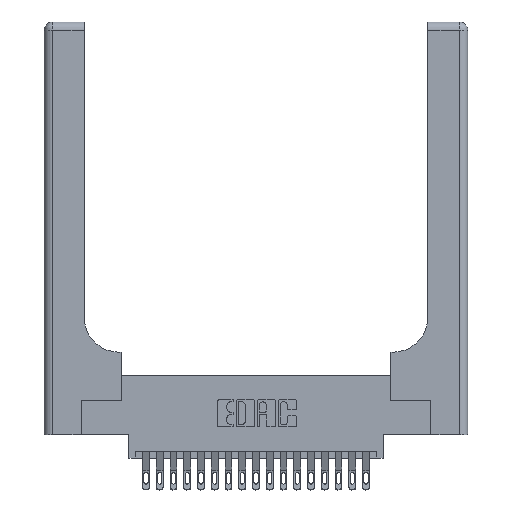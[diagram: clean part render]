
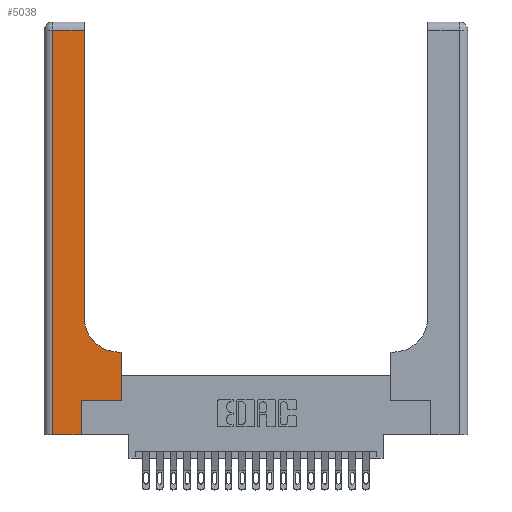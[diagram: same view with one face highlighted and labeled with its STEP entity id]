
A CAD part, top view. The second image highlights one B-rep face of the part: STEP entity #5038.
In plain terms, the highlighted planar face has unit normal (0, 0, 1).
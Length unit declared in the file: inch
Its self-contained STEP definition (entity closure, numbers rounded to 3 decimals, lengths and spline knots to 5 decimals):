
#271 = VERTEX_POINT ( 'NONE', #5505 ) ;
#707 = LINE ( 'NONE', #920, #3952 ) ;
#920 = CARTESIAN_POINT ( 'NONE',  ( 0., 2.94, 0.37 ) ) ;
#948 = LINE ( 'NONE', #12074, #3645 ) ;
#1036 = LINE ( 'NONE', #12148, #11002 ) ;
#1295 = CARTESIAN_POINT ( 'NONE',  ( 0.269, 0., 0.37 ) ) ;
#1308 = EDGE_CURVE ( 'NONE', #8733, #8761, #15321, .T. ) ;
#1400 = CIRCLE ( 'NONE', #7907, 0.25 ) ;
#1507 = CARTESIAN_POINT ( 'NONE',  ( 0.2915, 0.85, 0.37 ) ) ;
#1630 = ORIENTED_EDGE ( 'NONE', *, *, #9048, .T. ) ;
#2357 = DIRECTION ( 'NONE',  ( -1., 0., 0. ) ) ;
#2714 = VECTOR ( 'NONE', #3024, 39.37008 ) ;
#2720 = CARTESIAN_POINT ( 'NONE',  ( 0.5585, 0.6, 0.37 ) ) ;
#2778 = CARTESIAN_POINT ( 'NONE',  ( 0.269, 0.25, 0.37 ) ) ;
#2927 = CARTESIAN_POINT ( 'NONE',  ( 0.2915, 2.94, 0.37 ) ) ;
#3024 = DIRECTION ( 'NONE',  ( 0., 1., 0. ) ) ;
#3099 = VERTEX_POINT ( 'NONE', #20224 ) ;
#3645 = VECTOR ( 'NONE', #12151, 39.37008 ) ;
#3757 = DIRECTION ( 'NONE',  ( 1., 0., 0. ) ) ;
#3952 = VECTOR ( 'NONE', #19974, 39.37008 ) ;
#5038 = ADVANCED_FACE ( 'NONE', ( #20860 ), #10703, .F. ) ;
#5185 = DIRECTION ( 'NONE',  ( 0., 0., -1. ) ) ;
#5505 = CARTESIAN_POINT ( 'NONE',  ( 0.269, 0., 0.37 ) ) ;
#6190 = ORIENTED_EDGE ( 'NONE', *, *, #9986, .T. ) ;
#6917 = ORIENTED_EDGE ( 'NONE', *, *, #10793, .T. ) ;
#7112 = ORIENTED_EDGE ( 'NONE', *, *, #17414, .T. ) ;
#7198 = ORIENTED_EDGE ( 'NONE', *, *, #14333, .T. ) ;
#7817 = LINE ( 'NONE', #20428, #13221 ) ;
#7907 = AXIS2_PLACEMENT_3D ( 'NONE', #8858, #5185, #10287 ) ;
#8057 = ORIENTED_EDGE ( 'NONE', *, *, #1308, .T. ) ;
#8194 = AXIS2_PLACEMENT_3D ( 'NONE', #10933, #19510, #2357 ) ;
#8733 = VERTEX_POINT ( 'NONE', #13146 ) ;
#8761 = VERTEX_POINT ( 'NONE', #2720 ) ;
#8839 = VERTEX_POINT ( 'NONE', #1507 ) ;
#8858 = CARTESIAN_POINT ( 'NONE',  ( 0.5415, 0.85, 0.37 ) ) ;
#9048 = EDGE_CURVE ( 'NONE', #8839, #12609, #1036, .T. ) ;
#9986 = EDGE_CURVE ( 'NONE', #12609, #17768, #707, .T. ) ;
#10287 = DIRECTION ( 'NONE',  ( 1., 0., 0. ) ) ;
#10338 = ORIENTED_EDGE ( 'NONE', *, *, #17606, .T. ) ;
#10703 = PLANE ( 'NONE',  #8194 ) ;
#10793 = EDGE_CURVE ( 'NONE', #17768, #3099, #948, .T. ) ;
#10933 = CARTESIAN_POINT ( 'NONE',  ( 0., 3., 0.37 ) ) ;
#11002 = VECTOR ( 'NONE', #19029, 39.37008 ) ;
#11809 = VECTOR ( 'NONE', #13746, 39.37008 ) ;
#12074 = CARTESIAN_POINT ( 'NONE',  ( 0.06, 3., 0.37 ) ) ;
#12148 = CARTESIAN_POINT ( 'NONE',  ( 0.2915, 3., 0.37 ) ) ;
#12151 = DIRECTION ( 'NONE',  ( 0., -1., 0. ) ) ;
#12609 = VERTEX_POINT ( 'NONE', #2927 ) ;
#12983 = LINE ( 'NONE', #1295, #2714 ) ;
#13146 = CARTESIAN_POINT ( 'NONE',  ( 0.5585, 0.25, 0.37 ) ) ;
#13221 = VECTOR ( 'NONE', #17021, 39.37008 ) ;
#13746 = DIRECTION ( 'NONE',  ( 0., 1., 0. ) ) ;
#14045 = CARTESIAN_POINT ( 'NONE',  ( 0., 0., 0.37 ) ) ;
#14333 = EDGE_CURVE ( 'NONE', #3099, #271, #19948, .T. ) ;
#15143 = ORIENTED_EDGE ( 'NONE', *, *, #18635, .T. ) ;
#15321 = LINE ( 'NONE', #18801, #11809 ) ;
#15328 = VECTOR ( 'NONE', #3757, 39.37008 ) ;
#16232 = VERTEX_POINT ( 'NONE', #18431 ) ;
#17021 = DIRECTION ( 'NONE',  ( 1., 0., 0. ) ) ;
#17075 = LINE ( 'NONE', #20452, #22193 ) ;
#17414 = EDGE_CURVE ( 'NONE', #8761, #16232, #17075, .T. ) ;
#17606 = EDGE_CURVE ( 'NONE', #16232, #8839, #1400, .T. ) ;
#17768 = VERTEX_POINT ( 'NONE', #21169 ) ;
#17786 = EDGE_LOOP ( 'NONE', ( #1630, #6190, #6917, #7198, #15143, #21598, #8057, #7112, #10338 ) ) ;
#18431 = CARTESIAN_POINT ( 'NONE',  ( 0.5415, 0.6, 0.37 ) ) ;
#18635 = EDGE_CURVE ( 'NONE', #271, #19223, #12983, .T. ) ;
#18801 = CARTESIAN_POINT ( 'NONE',  ( 0.5585, 0.25, 0.37 ) ) ;
#19029 = DIRECTION ( 'NONE',  ( 0., 1., 0. ) ) ;
#19223 = VERTEX_POINT ( 'NONE', #2778 ) ;
#19510 = DIRECTION ( 'NONE',  ( 0., 0., -1. ) ) ;
#19948 = LINE ( 'NONE', #14045, #15328 ) ;
#19974 = DIRECTION ( 'NONE',  ( -1., 0., 0. ) ) ;
#20224 = CARTESIAN_POINT ( 'NONE',  ( 0.06, 0., 0.37 ) ) ;
#20428 = CARTESIAN_POINT ( 'NONE',  ( 0.269, 0.25, 0.37 ) ) ;
#20452 = CARTESIAN_POINT ( 'NONE',  ( 0.2915, 0.6, 0.37 ) ) ;
#20860 = FACE_OUTER_BOUND ( 'NONE', #17786, .T. ) ;
#21169 = CARTESIAN_POINT ( 'NONE',  ( 0.06, 2.94, 0.37 ) ) ;
#21516 = EDGE_CURVE ( 'NONE', #19223, #8733, #7817, .T. ) ;
#21598 = ORIENTED_EDGE ( 'NONE', *, *, #21516, .T. ) ;
#22078 = DIRECTION ( 'NONE',  ( -1., 0., 0. ) ) ;
#22193 = VECTOR ( 'NONE', #22078, 39.37008 ) ;
